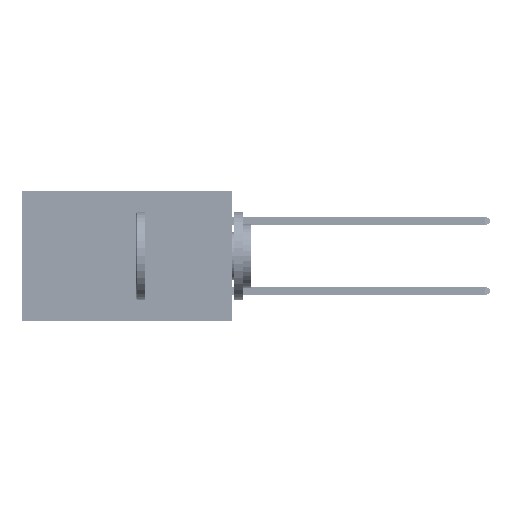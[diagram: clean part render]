
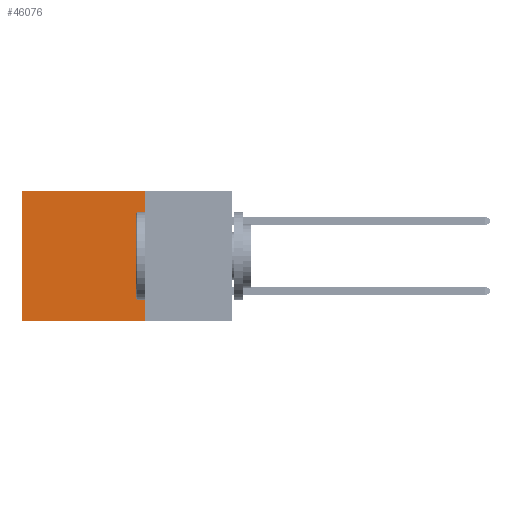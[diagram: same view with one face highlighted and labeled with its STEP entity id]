
A CAD part, left-side view. The second image highlights one B-rep face of the part: STEP entity #46076.
In plain terms, the highlighted planar face has unit normal (-1, 0, 0).
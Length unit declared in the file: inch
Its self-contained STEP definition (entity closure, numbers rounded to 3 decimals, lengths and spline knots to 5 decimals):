
#242 = VECTOR ( 'NONE', #36207, 39.37008 ) ;
#681 = ORIENTED_EDGE ( 'NONE', *, *, #25925, .T. ) ;
#3850 = EDGE_CURVE ( 'NONE', #38934, #24999, #3996, .T. ) ;
#3996 = LINE ( 'NONE', #11130, #13436 ) ;
#5053 = EDGE_LOOP ( 'NONE', ( #17531, #35812, #29079, #681 ) ) ;
#6222 = LINE ( 'NONE', #24395, #46918 ) ;
#6444 = EDGE_CURVE ( 'NONE', #24999, #40162, #6222, .T. ) ;
#7146 = LINE ( 'NONE', #32137, #242 ) ;
#7331 = DIRECTION ( 'NONE',  ( 1., 0., 0. ) ) ;
#11130 = CARTESIAN_POINT ( 'NONE',  ( 0.2875, 0.25, 0. ) ) ;
#12627 = DIRECTION ( 'NONE',  ( 0., 0., -1. ) ) ;
#13242 = CARTESIAN_POINT ( 'NONE',  ( 0.2875, 0.25, 0. ) ) ;
#13436 = VECTOR ( 'NONE', #47775, 39.37008 ) ;
#14613 = LINE ( 'NONE', #25043, #45832 ) ;
#17531 = ORIENTED_EDGE ( 'NONE', *, *, #52303, .T. ) ;
#19623 = CARTESIAN_POINT ( 'NONE',  ( 0.2875, 0.25, 0. ) ) ;
#23764 = PLANE ( 'NONE',  #24197 ) ;
#24197 = AXIS2_PLACEMENT_3D ( 'NONE', #19623, #7331, #52046 ) ;
#24395 = CARTESIAN_POINT ( 'NONE',  ( 0.2875, 0.25, -0.37 ) ) ;
#24999 = VERTEX_POINT ( 'NONE', #30818 ) ;
#25043 = CARTESIAN_POINT ( 'NONE',  ( 0.2875, 0.6, 0. ) ) ;
#25925 = EDGE_CURVE ( 'NONE', #38934, #39797, #7146, .T. ) ;
#28503 = DIRECTION ( 'NONE',  ( 0., 1., 0. ) ) ;
#29079 = ORIENTED_EDGE ( 'NONE', *, *, #3850, .F. ) ;
#30818 = CARTESIAN_POINT ( 'NONE',  ( 0.2875, 0.25, -0.37 ) ) ;
#32137 = CARTESIAN_POINT ( 'NONE',  ( 0.2875, 0.25, 0. ) ) ;
#34851 = CARTESIAN_POINT ( 'NONE',  ( 0.2875, 0.6, 0. ) ) ;
#35812 = ORIENTED_EDGE ( 'NONE', *, *, #6444, .F. ) ;
#36207 = DIRECTION ( 'NONE',  ( 0., 1., 0. ) ) ;
#38934 = VERTEX_POINT ( 'NONE', #13242 ) ;
#39797 = VERTEX_POINT ( 'NONE', #34851 ) ;
#40162 = VERTEX_POINT ( 'NONE', #48896 ) ;
#45816 = FACE_OUTER_BOUND ( 'NONE', #5053, .T. ) ;
#45832 = VECTOR ( 'NONE', #12627, 39.37008 ) ;
#46076 = ADVANCED_FACE ( 'NONE', ( #45816 ), #23764, .F. ) ;
#46918 = VECTOR ( 'NONE', #28503, 39.37008 ) ;
#47775 = DIRECTION ( 'NONE',  ( 0., 0., -1. ) ) ;
#48896 = CARTESIAN_POINT ( 'NONE',  ( 0.2875, 0.6, -0.37 ) ) ;
#52046 = DIRECTION ( 'NONE',  ( 0., 0., -1. ) ) ;
#52303 = EDGE_CURVE ( 'NONE', #39797, #40162, #14613, .T. ) ;
